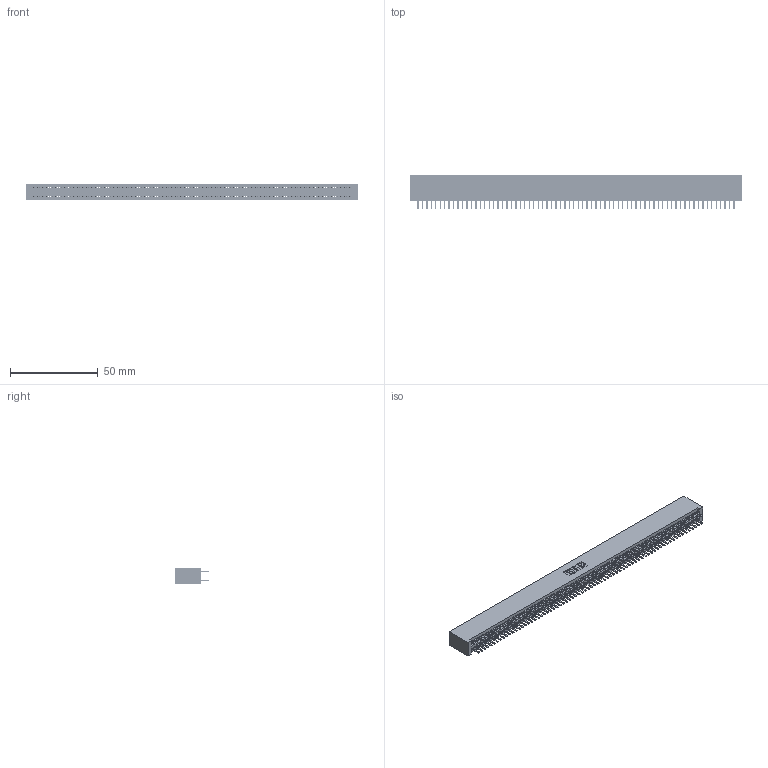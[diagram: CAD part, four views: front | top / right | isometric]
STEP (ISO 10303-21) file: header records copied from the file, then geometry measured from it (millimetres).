
FILE_DESCRIPTION (( 'STEP AP203' ), '1' );
FILE_NAME ('345-144-520-201.STEP', '2019-11-09T06:58:52', ( '' ), ( '' ), 'SwSTEP 2.0', 'SolidWorks 2016', '' );
FILE_SCHEMA (( 'CONFIG_CONTROL_DESIGN' ));
Length unit declared in the file: inch
Products named in the file (3): 345 Part_No Mounting Lugs; 345-144-520-201; 345-292-001_345-293-120
Assembly tree (145 placements, depth 2):
  345-144-520-201
    345 Part_No Mounting Lugs
    345-292-001_345-293-120  x144
Bounding box: 189.48 x 19.68 x 9.4 mm (x, y, z)
Volume: 19237.7 mm3; surface area: 29186.3 mm2
Topology: 145 solids, 145 shells, 7894 faces, 22925 edges, 14898 vertices
Faces by surface type: plane 5116, cylinder 2778
Entity records: 52291 total; most frequent: CARTESIAN_POINT 8748, ORIENTED_EDGE 8670, DIRECTION 7659, EDGE_CURVE 4335, LINE 3919, VECTOR 3919, VERTEX_POINT 2886, AXIS2_PLACEMENT_3D 1870
